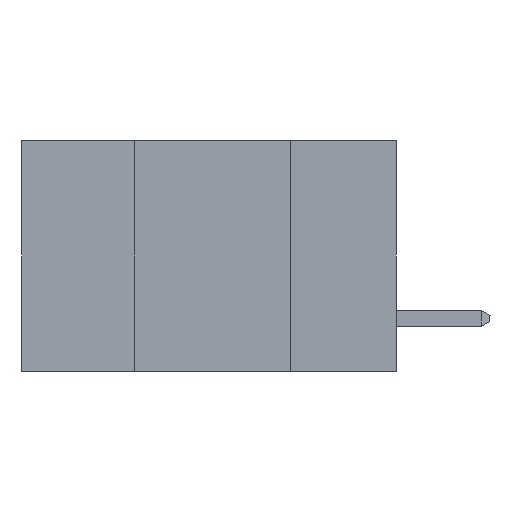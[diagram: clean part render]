
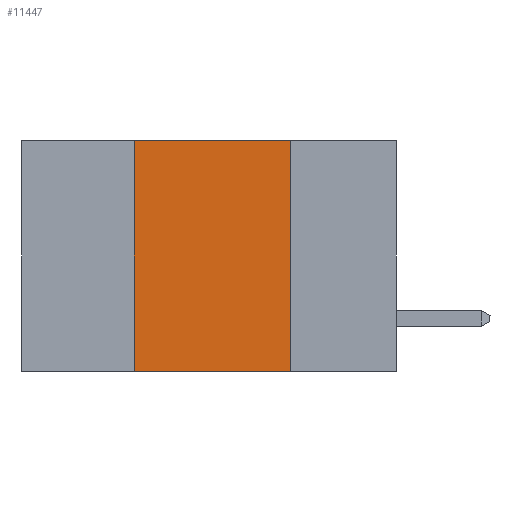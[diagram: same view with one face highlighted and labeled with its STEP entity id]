
A CAD part, left-side view. The second image highlights one B-rep face of the part: STEP entity #11447.
In plain terms, the highlighted planar face has unit normal (-1, 0, 0).
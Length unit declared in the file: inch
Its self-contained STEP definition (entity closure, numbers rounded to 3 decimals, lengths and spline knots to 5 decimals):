
#13 = EDGE_CURVE ( 'NONE', #1571, #489, #10750, .T. ) ;
#406 = CARTESIAN_POINT ( 'NONE',  ( 0., 0.42, -0.37 ) ) ;
#489 = VERTEX_POINT ( 'NONE', #10901 ) ;
#1571 = VERTEX_POINT ( 'NONE', #406 ) ;
#1789 = LINE ( 'NONE', #5067, #12385 ) ;
#2007 = DIRECTION ( 'NONE',  ( 1., 0., 0. ) ) ;
#2265 = DIRECTION ( 'NONE',  ( 0., 0., 1. ) ) ;
#2728 = CARTESIAN_POINT ( 'NONE',  ( 0., 0.42, -0.37 ) ) ;
#3002 = FACE_OUTER_BOUND ( 'NONE', #12571, .T. ) ;
#3560 = LINE ( 'NONE', #7932, #6039 ) ;
#4087 = ORIENTED_EDGE ( 'NONE', *, *, #6843, .T. ) ;
#4477 = VECTOR ( 'NONE', #11007, 39.37008 ) ;
#4983 = VECTOR ( 'NONE', #2265, 39.37008 ) ;
#4999 = AXIS2_PLACEMENT_3D ( 'NONE', #13764, #2007, #13582 ) ;
#5067 = CARTESIAN_POINT ( 'NONE',  ( 0., 0.6, 0. ) ) ;
#6039 = VECTOR ( 'NONE', #7858, 39.37008 ) ;
#6081 = EDGE_CURVE ( 'NONE', #8843, #8960, #3560, .T. ) ;
#6843 = EDGE_CURVE ( 'NONE', #1571, #8960, #6901, .T. ) ;
#6901 = LINE ( 'NONE', #12314, #4477 ) ;
#6902 = ORIENTED_EDGE ( 'NONE', *, *, #6081, .F. ) ;
#7089 = CARTESIAN_POINT ( 'NONE',  ( 0., 0.17, -0.37 ) ) ;
#7858 = DIRECTION ( 'NONE',  ( 0., 0., -1. ) ) ;
#7932 = CARTESIAN_POINT ( 'NONE',  ( 0., 0.17, -0.37 ) ) ;
#8125 = ORIENTED_EDGE ( 'NONE', *, *, #13, .F. ) ;
#8843 = VERTEX_POINT ( 'NONE', #13451 ) ;
#8960 = VERTEX_POINT ( 'NONE', #7089 ) ;
#9956 = EDGE_CURVE ( 'NONE', #489, #8843, #1789, .T. ) ;
#10371 = PLANE ( 'NONE',  #4999 ) ;
#10472 = ORIENTED_EDGE ( 'NONE', *, *, #9956, .F. ) ;
#10750 = LINE ( 'NONE', #2728, #4983 ) ;
#10901 = CARTESIAN_POINT ( 'NONE',  ( 0., 0.42, 0. ) ) ;
#11007 = DIRECTION ( 'NONE',  ( 0., -1., 0. ) ) ;
#11447 = ADVANCED_FACE ( 'NONE', ( #3002 ), #10371, .F. ) ;
#11507 = DIRECTION ( 'NONE',  ( 0., -1., 0. ) ) ;
#12314 = CARTESIAN_POINT ( 'NONE',  ( 0., 0.6, -0.37 ) ) ;
#12385 = VECTOR ( 'NONE', #11507, 39.37008 ) ;
#12571 = EDGE_LOOP ( 'NONE', ( #6902, #10472, #8125, #4087 ) ) ;
#13451 = CARTESIAN_POINT ( 'NONE',  ( 0., 0.17, 0. ) ) ;
#13582 = DIRECTION ( 'NONE',  ( 0., 0., -1. ) ) ;
#13764 = CARTESIAN_POINT ( 'NONE',  ( 0., 0.6, 0. ) ) ;
